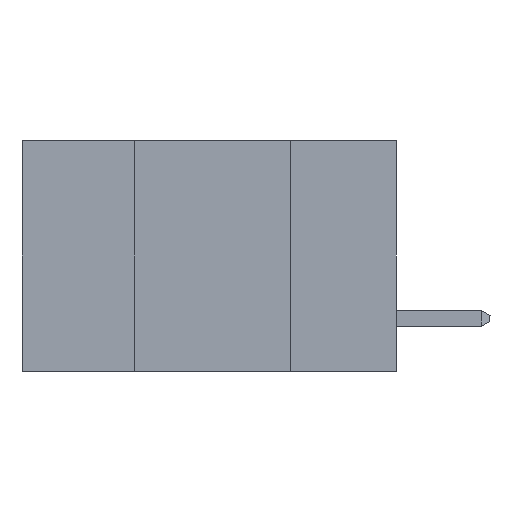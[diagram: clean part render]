
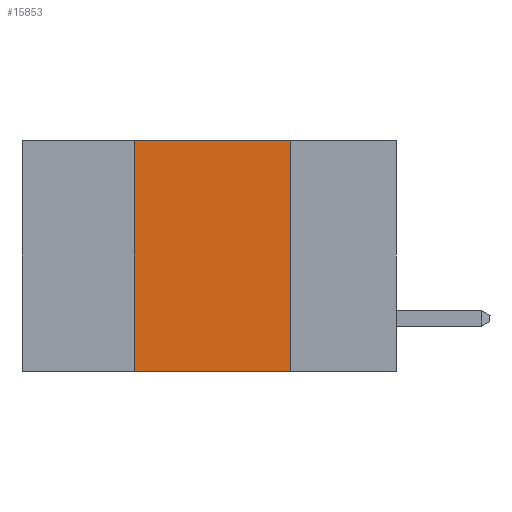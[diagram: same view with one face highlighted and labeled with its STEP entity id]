
A CAD part, left-side view. The second image highlights one B-rep face of the part: STEP entity #15853.
In plain terms, the highlighted planar face has unit normal (-1, 0, 0).
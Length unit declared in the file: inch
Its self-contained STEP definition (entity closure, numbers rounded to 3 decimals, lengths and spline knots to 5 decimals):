
#721 = CARTESIAN_POINT ( 'NONE',  ( 0., 0.17, 0. ) ) ;
#922 = CARTESIAN_POINT ( 'NONE',  ( 0., 0.6, -0.37 ) ) ;
#2283 = DIRECTION ( 'NONE',  ( 0., -1., 0. ) ) ;
#2491 = LINE ( 'NONE', #922, #15629 ) ;
#2654 = LINE ( 'NONE', #13283, #6283 ) ;
#3460 = FACE_OUTER_BOUND ( 'NONE', #15636, .T. ) ;
#3710 = LINE ( 'NONE', #4708, #10737 ) ;
#3774 = CARTESIAN_POINT ( 'NONE',  ( 0., 0.42, -0.37 ) ) ;
#3851 = VERTEX_POINT ( 'NONE', #10649 ) ;
#4708 = CARTESIAN_POINT ( 'NONE',  ( 0., 0.17, -0.37 ) ) ;
#5473 = VECTOR ( 'NONE', #9654, 39.37008 ) ;
#5499 = DIRECTION ( 'NONE',  ( 0., 0., 1. ) ) ;
#5744 = VERTEX_POINT ( 'NONE', #13823 ) ;
#5887 = DIRECTION ( 'NONE',  ( 1., 0., 0. ) ) ;
#6283 = VECTOR ( 'NONE', #5499, 39.37008 ) ;
#7098 = CARTESIAN_POINT ( 'NONE',  ( 0., 0.6, 0. ) ) ;
#7189 = VERTEX_POINT ( 'NONE', #3774 ) ;
#7937 = ORIENTED_EDGE ( 'NONE', *, *, #11327, .T. ) ;
#8159 = EDGE_CURVE ( 'NONE', #3851, #14032, #8935, .T. ) ;
#8434 = CARTESIAN_POINT ( 'NONE',  ( 0., 0.6, 0. ) ) ;
#8935 = LINE ( 'NONE', #7098, #5473 ) ;
#9654 = DIRECTION ( 'NONE',  ( 0., -1., 0. ) ) ;
#9923 = DIRECTION ( 'NONE',  ( 0., 0., -1. ) ) ;
#10649 = CARTESIAN_POINT ( 'NONE',  ( 0., 0.42, 0. ) ) ;
#10737 = VECTOR ( 'NONE', #9923, 39.37008 ) ;
#11244 = ORIENTED_EDGE ( 'NONE', *, *, #8159, .F. ) ;
#11327 = EDGE_CURVE ( 'NONE', #7189, #5744, #2491, .T. ) ;
#11433 = ORIENTED_EDGE ( 'NONE', *, *, #12764, .F. ) ;
#12383 = PLANE ( 'NONE',  #15842 ) ;
#12451 = ORIENTED_EDGE ( 'NONE', *, *, #12528, .F. ) ;
#12528 = EDGE_CURVE ( 'NONE', #14032, #5744, #3710, .T. ) ;
#12764 = EDGE_CURVE ( 'NONE', #7189, #3851, #2654, .T. ) ;
#13283 = CARTESIAN_POINT ( 'NONE',  ( 0., 0.42, -0.37 ) ) ;
#13823 = CARTESIAN_POINT ( 'NONE',  ( 0., 0.17, -0.37 ) ) ;
#14032 = VERTEX_POINT ( 'NONE', #721 ) ;
#14938 = DIRECTION ( 'NONE',  ( 0., 0., -1. ) ) ;
#15629 = VECTOR ( 'NONE', #2283, 39.37008 ) ;
#15636 = EDGE_LOOP ( 'NONE', ( #12451, #11244, #11433, #7937 ) ) ;
#15842 = AXIS2_PLACEMENT_3D ( 'NONE', #8434, #5887, #14938 ) ;
#15853 = ADVANCED_FACE ( 'NONE', ( #3460 ), #12383, .F. ) ;
